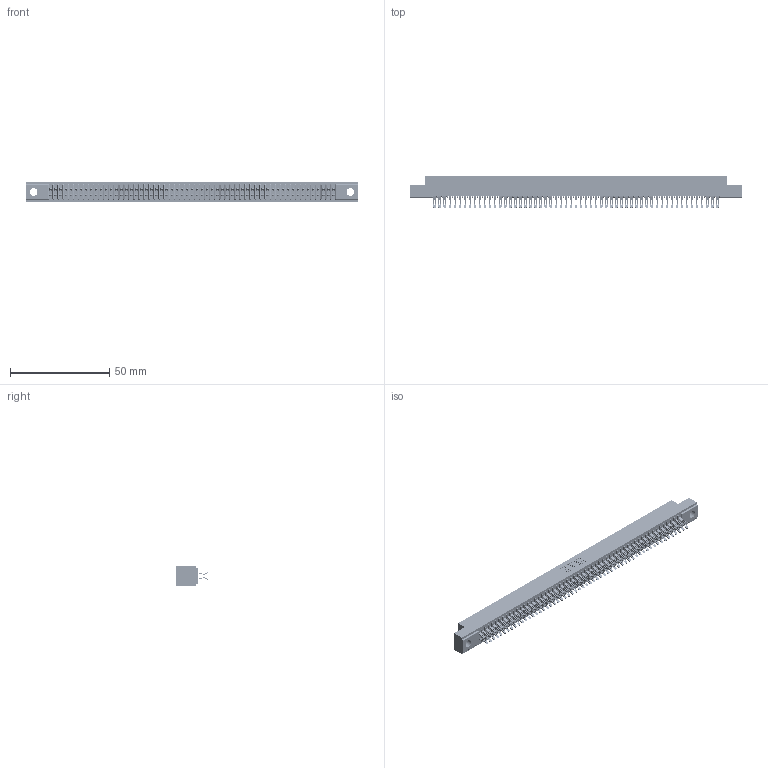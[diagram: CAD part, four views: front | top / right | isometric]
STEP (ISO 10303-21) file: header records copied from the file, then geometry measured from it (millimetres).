
FILE_DESCRIPTION (( 'STEP AP203' ), '1' );
FILE_NAME ('391-114-555-204.STEP', '2018-08-09T22:49:06', ( '' ), ( '' ), 'SwSTEP 2.0', 'SolidWorks 2016', '' );
FILE_SCHEMA (( 'CONFIG_CONTROL_DESIGN' ));
Length unit declared in the file: inch
Products named in the file (3): 341 Part_.156 (3.96) Dia Mounting Holes; 341-292-001_341-292-155; 391-114-555-204
Assembly tree (115 placements, depth 2):
  391-114-555-204
    341 Part_.156 (3.96) Dia Mounting Holes
    341-292-001_341-292-155  x114
Bounding box: 167 x 16.31 x 10.16 mm (x, y, z)
Volume: 12384.7 mm3; surface area: 23274.7 mm2
Topology: 115 solids, 115 shells, 9022 faces, 26971 edges, 17558 vertices
Faces by surface type: plane 4870, cylinder 3924, sphere 116, torus 112
Entity records: 67872 total; most frequent: CARTESIAN_POINT 11303, ORIENTED_EDGE 11222, DIRECTION 10941, EDGE_CURVE 5611, VECTOR 4541, LINE 4541, VERTEX_POINT 3546, AXIS2_PLACEMENT_3D 3200
